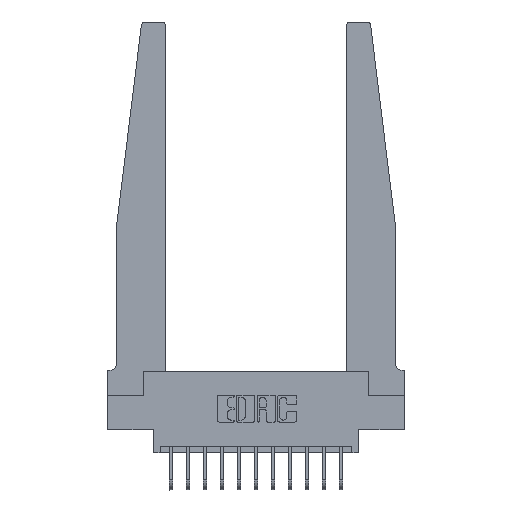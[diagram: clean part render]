
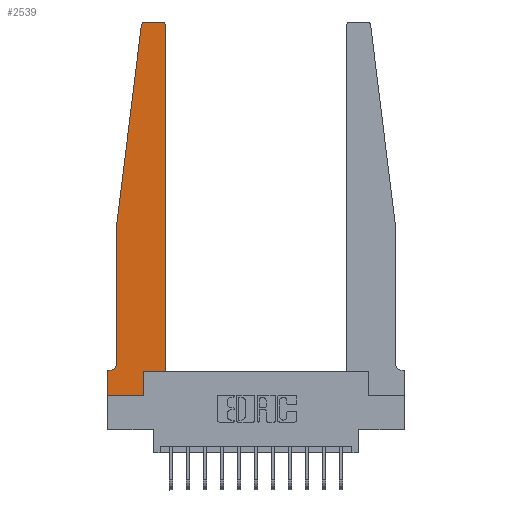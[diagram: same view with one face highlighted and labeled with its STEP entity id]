
A CAD part, top view. The second image highlights one B-rep face of the part: STEP entity #2539.
In plain terms, the highlighted planar face has unit normal (0, 0, 1).
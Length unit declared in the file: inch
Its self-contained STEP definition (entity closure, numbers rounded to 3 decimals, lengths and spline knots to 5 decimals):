
#8 = LINE ( 'NONE', #4067, #10882 ) ;
#38 = ORIENTED_EDGE ( 'NONE', *, *, #6448, .T. ) ;
#224 = AXIS2_PLACEMENT_3D ( 'NONE', #15828, #1835, #8996 ) ;
#360 = ORIENTED_EDGE ( 'NONE', *, *, #2437, .T. ) ;
#405 = DIRECTION ( 'NONE',  ( -0.122, -0.992, 0. ) ) ;
#413 = VECTOR ( 'NONE', #1062, 39.37008 ) ;
#524 = DIRECTION ( 'NONE',  ( -1., 0., 0. ) ) ;
#1062 = DIRECTION ( 'NONE',  ( 1., 0., 0. ) ) ;
#1236 = VERTEX_POINT ( 'NONE', #12471 ) ;
#1249 = CARTESIAN_POINT ( 'NONE',  ( 0.065, 0.2375, 0.37 ) ) ;
#1679 = EDGE_CURVE ( 'NONE', #1236, #10587, #13186, .T. ) ;
#1700 = VECTOR ( 'NONE', #405, 39.37008 ) ;
#1835 = DIRECTION ( 'NONE',  ( 0., 0., -1. ) ) ;
#2091 = CIRCLE ( 'NONE', #224, 0.05 ) ;
#2245 = DIRECTION ( 'NONE',  ( 0., 1., 0. ) ) ;
#2266 = EDGE_CURVE ( 'NONE', #5644, #14338, #2091, .T. ) ;
#2437 = EDGE_CURVE ( 'NONE', #10587, #14912, #7139, .T. ) ;
#2457 = CARTESIAN_POINT ( 'NONE',  ( 0., 0., 0.37 ) ) ;
#2539 = ADVANCED_FACE ( 'NONE', ( #12633 ), #10222, .T. ) ;
#2583 = CARTESIAN_POINT ( 'NONE',  ( 0.015, 0.1875, 0.37 ) ) ;
#2688 = EDGE_CURVE ( 'NONE', #4184, #8278, #7972, .T. ) ;
#3037 = CARTESIAN_POINT ( 'NONE',  ( 0.425, 0.18, 0.37 ) ) ;
#3550 = CARTESIAN_POINT ( 'NONE',  ( 0.27653, 2.72, 0.37 ) ) ;
#3621 = CARTESIAN_POINT ( 'NONE',  ( 0.24675, 2.72367, 0.37 ) ) ;
#3638 = DIRECTION ( 'NONE',  ( 0., -1., 0. ) ) ;
#3784 = ORIENTED_EDGE ( 'NONE', *, *, #5689, .T. ) ;
#4066 = ORIENTED_EDGE ( 'NONE', *, *, #2688, .T. ) ;
#4067 = CARTESIAN_POINT ( 'NONE',  ( 0.065, 0.1875, 0.37 ) ) ;
#4093 = VERTEX_POINT ( 'NONE', #11254 ) ;
#4184 = VERTEX_POINT ( 'NONE', #3621 ) ;
#4248 = CARTESIAN_POINT ( 'NONE',  ( 0., 0.1875, 0.37 ) ) ;
#4381 = CARTESIAN_POINT ( 'NONE',  ( 0.425, 2.72, 0.37 ) ) ;
#4649 = EDGE_CURVE ( 'NONE', #14912, #9905, #7385, .T. ) ;
#4867 = DIRECTION ( 'NONE',  ( 1., 0., 0. ) ) ;
#4899 = CARTESIAN_POINT ( 'NONE',  ( 0.065, 1.25, 0.37 ) ) ;
#5327 = EDGE_CURVE ( 'NONE', #4093, #1236, #11895, .T. ) ;
#5399 = DIRECTION ( 'NONE',  ( 1., 0., 0. ) ) ;
#5612 = AXIS2_PLACEMENT_3D ( 'NONE', #3550, #6050, #11304 ) ;
#5644 = VERTEX_POINT ( 'NONE', #1249 ) ;
#5689 = EDGE_CURVE ( 'NONE', #7379, #5854, #9039, .T. ) ;
#5792 = LINE ( 'NONE', #2457, #413 ) ;
#5854 = VERTEX_POINT ( 'NONE', #14495 ) ;
#6050 = DIRECTION ( 'NONE',  ( 0., 0., 1. ) ) ;
#6070 = CARTESIAN_POINT ( 'NONE',  ( 0.425, 0.18, 0.37 ) ) ;
#6221 = LINE ( 'NONE', #4899, #6617 ) ;
#6308 = CARTESIAN_POINT ( 'NONE',  ( 0., 0.1875, 0.37 ) ) ;
#6347 = AXIS2_PLACEMENT_3D ( 'NONE', #6308, #7815, #15093 ) ;
#6448 = EDGE_CURVE ( 'NONE', #8278, #5644, #6221, .T. ) ;
#6495 = ORIENTED_EDGE ( 'NONE', *, *, #14849, .T. ) ;
#6617 = VECTOR ( 'NONE', #3638, 39.37008 ) ;
#6752 = EDGE_LOOP ( 'NONE', ( #12223, #14276, #4066, #38, #11673, #6495, #3784, #14887, #10337, #10650, #360, #13024 ) ) ;
#7139 = LINE ( 'NONE', #6070, #16420 ) ;
#7379 = VERTEX_POINT ( 'NONE', #4248 ) ;
#7385 = CIRCLE ( 'NONE', #11402, 0.03 ) ;
#7815 = DIRECTION ( 'NONE',  ( 0., 0., 1. ) ) ;
#7906 = CARTESIAN_POINT ( 'NONE',  ( 0.2605, 0.18, 0.37 ) ) ;
#7972 = LINE ( 'NONE', #11803, #1700 ) ;
#8278 = VERTEX_POINT ( 'NONE', #10784 ) ;
#8451 = VECTOR ( 'NONE', #524, 39.37008 ) ;
#8509 = CIRCLE ( 'NONE', #5612, 0.03 ) ;
#8996 = DIRECTION ( 'NONE',  ( -1., 0., 0. ) ) ;
#9039 = LINE ( 'NONE', #9192, #11986 ) ;
#9192 = CARTESIAN_POINT ( 'NONE',  ( 0., 0., 0.37 ) ) ;
#9322 = CARTESIAN_POINT ( 'NONE',  ( 0.27653, 2.75, 0.37 ) ) ;
#9905 = VERTEX_POINT ( 'NONE', #12667 ) ;
#10222 = PLANE ( 'NONE',  #6347 ) ;
#10337 = ORIENTED_EDGE ( 'NONE', *, *, #5327, .T. ) ;
#10550 = DIRECTION ( 'NONE',  ( 0., -1., 0. ) ) ;
#10587 = VERTEX_POINT ( 'NONE', #3037 ) ;
#10650 = ORIENTED_EDGE ( 'NONE', *, *, #1679, .T. ) ;
#10684 = EDGE_CURVE ( 'NONE', #5854, #4093, #5792, .T. ) ;
#10784 = CARTESIAN_POINT ( 'NONE',  ( 0.065, 1.25, 0.37 ) ) ;
#10882 = VECTOR ( 'NONE', #13936, 39.37008 ) ;
#11203 = CARTESIAN_POINT ( 'NONE',  ( 0.395, 2.72, 0.37 ) ) ;
#11254 = CARTESIAN_POINT ( 'NONE',  ( 0.2605, 0., 0.37 ) ) ;
#11304 = DIRECTION ( 'NONE',  ( 1., 0., 0. ) ) ;
#11402 = AXIS2_PLACEMENT_3D ( 'NONE', #11203, #16214, #4867 ) ;
#11673 = ORIENTED_EDGE ( 'NONE', *, *, #2266, .T. ) ;
#11801 = CARTESIAN_POINT ( 'NONE',  ( 0.425, 0.18, 0.37 ) ) ;
#11803 = CARTESIAN_POINT ( 'NONE',  ( 0.065, 1.25, 0.37 ) ) ;
#11895 = LINE ( 'NONE', #7906, #14803 ) ;
#11897 = CARTESIAN_POINT ( 'NONE',  ( 0.25, 2.75, 0.37 ) ) ;
#11986 = VECTOR ( 'NONE', #10550, 39.37008 ) ;
#12223 = ORIENTED_EDGE ( 'NONE', *, *, #14491, .T. ) ;
#12471 = CARTESIAN_POINT ( 'NONE',  ( 0.2605, 0.18, 0.37 ) ) ;
#12633 = FACE_OUTER_BOUND ( 'NONE', #6752, .T. ) ;
#12667 = CARTESIAN_POINT ( 'NONE',  ( 0.395, 2.75, 0.37 ) ) ;
#13024 = ORIENTED_EDGE ( 'NONE', *, *, #4649, .T. ) ;
#13186 = LINE ( 'NONE', #11801, #14518 ) ;
#13936 = DIRECTION ( 'NONE',  ( -1., 0., 0. ) ) ;
#14276 = ORIENTED_EDGE ( 'NONE', *, *, #16387, .T. ) ;
#14338 = VERTEX_POINT ( 'NONE', #2583 ) ;
#14367 = DIRECTION ( 'NONE',  ( 0., 1., 0. ) ) ;
#14491 = EDGE_CURVE ( 'NONE', #9905, #15221, #15920, .T. ) ;
#14495 = CARTESIAN_POINT ( 'NONE',  ( 0., 0., 0.37 ) ) ;
#14518 = VECTOR ( 'NONE', #5399, 39.37008 ) ;
#14803 = VECTOR ( 'NONE', #14367, 39.37008 ) ;
#14849 = EDGE_CURVE ( 'NONE', #14338, #7379, #8, .T. ) ;
#14887 = ORIENTED_EDGE ( 'NONE', *, *, #10684, .T. ) ;
#14912 = VERTEX_POINT ( 'NONE', #4381 ) ;
#15093 = DIRECTION ( 'NONE',  ( 1., 0., 0. ) ) ;
#15221 = VERTEX_POINT ( 'NONE', #9322 ) ;
#15828 = CARTESIAN_POINT ( 'NONE',  ( 0.015, 0.2375, 0.37 ) ) ;
#15920 = LINE ( 'NONE', #11897, #8451 ) ;
#16214 = DIRECTION ( 'NONE',  ( 0., 0., 1. ) ) ;
#16387 = EDGE_CURVE ( 'NONE', #15221, #4184, #8509, .T. ) ;
#16420 = VECTOR ( 'NONE', #2245, 39.37008 ) ;
